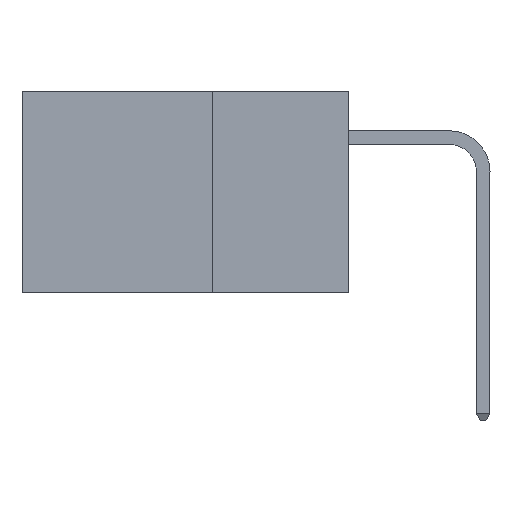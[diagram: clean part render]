
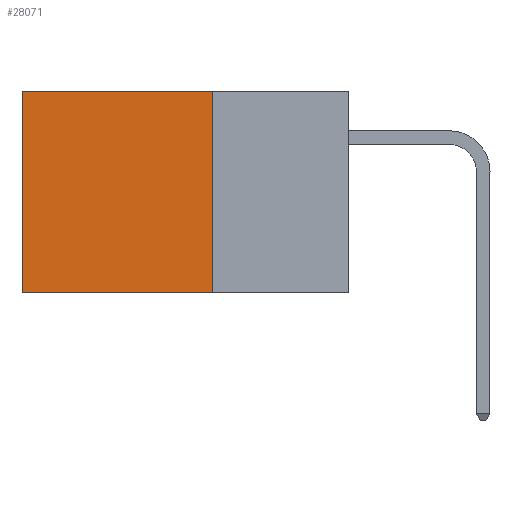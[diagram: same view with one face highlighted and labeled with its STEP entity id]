
A CAD part, left-side view. The second image highlights one B-rep face of the part: STEP entity #28071.
In plain terms, the highlighted planar face has unit normal (-1, 0, 0).
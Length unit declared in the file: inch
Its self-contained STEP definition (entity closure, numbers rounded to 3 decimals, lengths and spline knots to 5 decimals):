
#309 = CARTESIAN_POINT ( 'NONE',  ( 0.2875, 0.25, 0. ) ) ;
#1082 = DIRECTION ( 'NONE',  ( 0., 1., 0. ) ) ;
#1551 = VECTOR ( 'NONE', #20278, 39.37008 ) ;
#2602 = FACE_OUTER_BOUND ( 'NONE', #34780, .T. ) ;
#2974 = VECTOR ( 'NONE', #3514, 39.37008 ) ;
#3163 = CARTESIAN_POINT ( 'NONE',  ( 0.2875, 0.25, 0. ) ) ;
#3514 = DIRECTION ( 'NONE',  ( 0., 1., 0. ) ) ;
#6081 = DIRECTION ( 'NONE',  ( 0., 0., -1. ) ) ;
#6675 = EDGE_CURVE ( 'NONE', #20685, #19463, #18175, .T. ) ;
#8370 = LINE ( 'NONE', #309, #1551 ) ;
#8626 = CARTESIAN_POINT ( 'NONE',  ( 0.2875, 0.6, -0.37 ) ) ;
#9487 = VERTEX_POINT ( 'NONE', #22855 ) ;
#9583 = VECTOR ( 'NONE', #12791, 39.37008 ) ;
#10375 = ORIENTED_EDGE ( 'NONE', *, *, #16242, .T. ) ;
#11023 = VERTEX_POINT ( 'NONE', #15668 ) ;
#11577 = EDGE_CURVE ( 'NONE', #11023, #9487, #23853, .T. ) ;
#12791 = DIRECTION ( 'NONE',  ( 0., 0., -1. ) ) ;
#13404 = ORIENTED_EDGE ( 'NONE', *, *, #14110, .F. ) ;
#14110 = EDGE_CURVE ( 'NONE', #11023, #20685, #8370, .T. ) ;
#14517 = PLANE ( 'NONE',  #31666 ) ;
#15668 = CARTESIAN_POINT ( 'NONE',  ( 0.2875, 0.25, 0. ) ) ;
#16242 = EDGE_CURVE ( 'NONE', #9487, #19463, #17140, .T. ) ;
#17140 = LINE ( 'NONE', #23855, #9583 ) ;
#17450 = VECTOR ( 'NONE', #1082, 39.37008 ) ;
#17650 = ORIENTED_EDGE ( 'NONE', *, *, #11577, .T. ) ;
#18175 = LINE ( 'NONE', #23231, #2974 ) ;
#19463 = VERTEX_POINT ( 'NONE', #8626 ) ;
#20278 = DIRECTION ( 'NONE',  ( 0., 0., -1. ) ) ;
#20685 = VERTEX_POINT ( 'NONE', #36073 ) ;
#20962 = CARTESIAN_POINT ( 'NONE',  ( 0.2875, 0.25, 0. ) ) ;
#21292 = ORIENTED_EDGE ( 'NONE', *, *, #6675, .F. ) ;
#22855 = CARTESIAN_POINT ( 'NONE',  ( 0.2875, 0.6, 0. ) ) ;
#22886 = DIRECTION ( 'NONE',  ( 1., 0., 0. ) ) ;
#23231 = CARTESIAN_POINT ( 'NONE',  ( 0.2875, 0.25, -0.37 ) ) ;
#23853 = LINE ( 'NONE', #20962, #17450 ) ;
#23855 = CARTESIAN_POINT ( 'NONE',  ( 0.2875, 0.6, 0. ) ) ;
#28071 = ADVANCED_FACE ( 'NONE', ( #2602 ), #14517, .F. ) ;
#31666 = AXIS2_PLACEMENT_3D ( 'NONE', #3163, #22886, #6081 ) ;
#34780 = EDGE_LOOP ( 'NONE', ( #10375, #21292, #13404, #17650 ) ) ;
#36073 = CARTESIAN_POINT ( 'NONE',  ( 0.2875, 0.25, -0.37 ) ) ;
